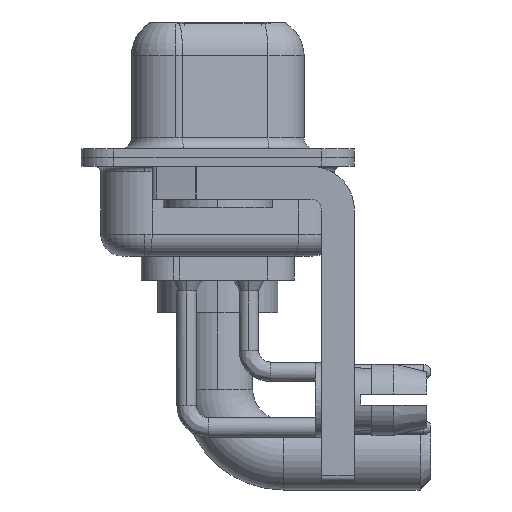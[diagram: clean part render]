
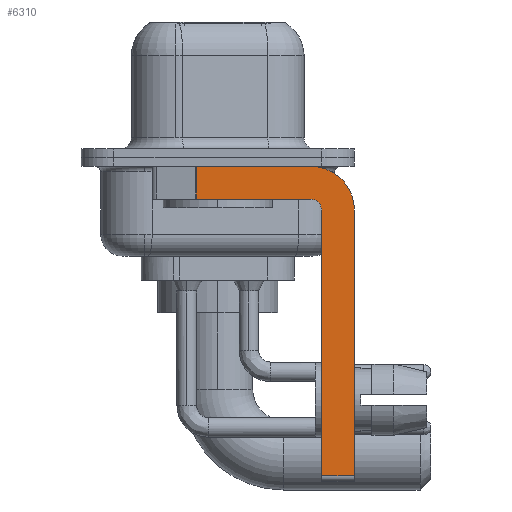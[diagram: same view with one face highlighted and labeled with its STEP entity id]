
A CAD part, left-side view. The second image highlights one B-rep face of the part: STEP entity #6310.
In plain terms, the highlighted planar face has unit normal (-1, 0, 0).
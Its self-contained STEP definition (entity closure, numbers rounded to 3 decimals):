
#52 = ORIENTED_EDGE ( 'NONE', *, *, #2772, .T. ) ;
#444 = CARTESIAN_POINT ( 'NONE',  ( -2.9, -6.25, -2.4 ) ) ;
#616 = FACE_OUTER_BOUND ( 'NONE', #15058, .T. ) ;
#1343 = VERTEX_POINT ( 'NONE', #12775 ) ;
#1422 = ORIENTED_EDGE ( 'NONE', *, *, #4371, .F. ) ;
#1679 = VECTOR ( 'NONE', #19840, 1000. ) ;
#2304 = CARTESIAN_POINT ( 'NONE',  ( -2.9, -4.25, -1.9 ) ) ;
#2448 = VECTOR ( 'NONE', #9069, 1000. ) ;
#2618 = EDGE_CURVE ( 'NONE', #14905, #4144, #6214, .T. ) ;
#2772 = EDGE_CURVE ( 'NONE', #11552, #1343, #19969, .T. ) ;
#3260 = VERTEX_POINT ( 'NONE', #4488 ) ;
#3313 = EDGE_CURVE ( 'NONE', #3260, #14905, #4277, .T. ) ;
#3354 = DIRECTION ( 'NONE',  ( 0., 0., 1. ) ) ;
#3613 = EDGE_CURVE ( 'NONE', #3260, #9450, #8724, .T. ) ;
#3883 = VERTEX_POINT ( 'NONE', #17448 ) ;
#4144 = VERTEX_POINT ( 'NONE', #2304 ) ;
#4277 = LINE ( 'NONE', #9496, #2448 ) ;
#4371 = EDGE_CURVE ( 'NONE', #11552, #3883, #14835, .T. ) ;
#4414 = CARTESIAN_POINT ( 'NONE',  ( -2.9, -4.25, -2.4 ) ) ;
#4488 = CARTESIAN_POINT ( 'NONE',  ( -2.9, -4.75, -14.55 ) ) ;
#5622 = DIRECTION ( 'NONE',  ( 1., 0., 0. ) ) ;
#5794 = DIRECTION ( 'NONE',  ( 0., 0., -1. ) ) ;
#6004 = DIRECTION ( 'NONE',  ( 1., 0., 0. ) ) ;
#6214 = CIRCLE ( 'NONE', #9983, 0.5 ) ;
#6310 = ADVANCED_FACE ( 'NONE', ( #616 ), #15322, .F. ) ;
#6884 = CIRCLE ( 'NONE', #10981, 2. ) ;
#6923 = CARTESIAN_POINT ( 'NONE',  ( -2.9, -4.25, -14.55 ) ) ;
#7077 = ORIENTED_EDGE ( 'NONE', *, *, #3613, .T. ) ;
#7244 = VECTOR ( 'NONE', #10438, 1000. ) ;
#7330 = ORIENTED_EDGE ( 'NONE', *, *, #9206, .F. ) ;
#8724 = LINE ( 'NONE', #6923, #7244 ) ;
#8840 = DIRECTION ( 'NONE',  ( 0., 1., 0. ) ) ;
#8887 = CARTESIAN_POINT ( 'NONE',  ( -2.9, 0.978, -1.9 ) ) ;
#8896 = VERTEX_POINT ( 'NONE', #14082 ) ;
#9069 = DIRECTION ( 'NONE',  ( 0., 0., 1. ) ) ;
#9155 = CARTESIAN_POINT ( 'NONE',  ( -2.9, -4.25, -1.9 ) ) ;
#9206 = EDGE_CURVE ( 'NONE', #8896, #9450, #13330, .T. ) ;
#9400 = ORIENTED_EDGE ( 'NONE', *, *, #2618, .F. ) ;
#9450 = VERTEX_POINT ( 'NONE', #11300 ) ;
#9496 = CARTESIAN_POINT ( 'NONE',  ( -2.9, -4.75, -14.8 ) ) ;
#9983 = AXIS2_PLACEMENT_3D ( 'NONE', #18160, #16571, #3354 ) ;
#10438 = DIRECTION ( 'NONE',  ( 0., -1., 0. ) ) ;
#10597 = VECTOR ( 'NONE', #12734, 1000. ) ;
#10636 = CARTESIAN_POINT ( 'NONE',  ( -2.9, 0.978, -0.4 ) ) ;
#10662 = LINE ( 'NONE', #9155, #10813 ) ;
#10813 = VECTOR ( 'NONE', #8840, 1000. ) ;
#10981 = AXIS2_PLACEMENT_3D ( 'NONE', #4414, #6004, #12499 ) ;
#11300 = CARTESIAN_POINT ( 'NONE',  ( -2.9, -6.25, -14.55 ) ) ;
#11552 = VERTEX_POINT ( 'NONE', #10636 ) ;
#11957 = ORIENTED_EDGE ( 'NONE', *, *, #20001, .F. ) ;
#12007 = EDGE_CURVE ( 'NONE', #3883, #8896, #6884, .T. ) ;
#12121 = DIRECTION ( 'NONE',  ( 0., 0., -1. ) ) ;
#12499 = DIRECTION ( 'NONE',  ( 0., 0., -1. ) ) ;
#12520 = AXIS2_PLACEMENT_3D ( 'NONE', #20217, #5622, #12121 ) ;
#12734 = DIRECTION ( 'NONE',  ( 0., -1., 0. ) ) ;
#12775 = CARTESIAN_POINT ( 'NONE',  ( -2.9, 0.978, -1.9 ) ) ;
#13330 = LINE ( 'NONE', #444, #1679 ) ;
#14082 = CARTESIAN_POINT ( 'NONE',  ( -2.9, -6.25, -2.4 ) ) ;
#14340 = ORIENTED_EDGE ( 'NONE', *, *, #12007, .F. ) ;
#14835 = LINE ( 'NONE', #19847, #10597 ) ;
#14905 = VERTEX_POINT ( 'NONE', #15834 ) ;
#15058 = EDGE_LOOP ( 'NONE', ( #1422, #52, #11957, #9400, #15557, #7077, #7330, #14340 ) ) ;
#15322 = PLANE ( 'NONE',  #12520 ) ;
#15557 = ORIENTED_EDGE ( 'NONE', *, *, #3313, .F. ) ;
#15834 = CARTESIAN_POINT ( 'NONE',  ( -2.9, -4.75, -2.4 ) ) ;
#16571 = DIRECTION ( 'NONE',  ( -1., 0., 0. ) ) ;
#17448 = CARTESIAN_POINT ( 'NONE',  ( -2.9, -4.25, -0.4 ) ) ;
#18160 = CARTESIAN_POINT ( 'NONE',  ( -2.9, -4.25, -2.4 ) ) ;
#19840 = DIRECTION ( 'NONE',  ( 0., 0., -1. ) ) ;
#19847 = CARTESIAN_POINT ( 'NONE',  ( -2.9, 3., -0.4 ) ) ;
#19860 = VECTOR ( 'NONE', #5794, 1000. ) ;
#19969 = LINE ( 'NONE', #8887, #19860 ) ;
#20001 = EDGE_CURVE ( 'NONE', #4144, #1343, #10662, .T. ) ;
#20217 = CARTESIAN_POINT ( 'NONE',  ( -2.9, -4.25, -2.4 ) ) ;
